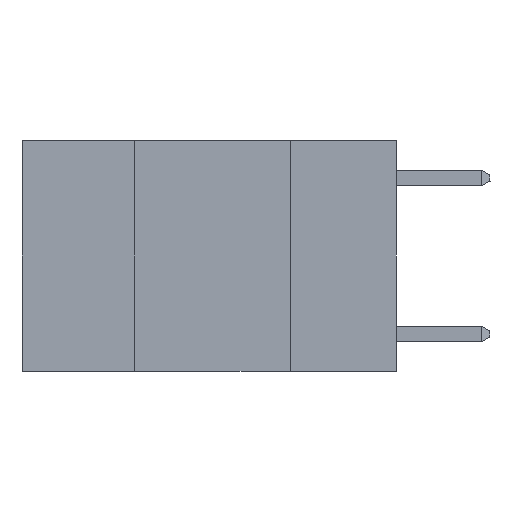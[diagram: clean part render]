
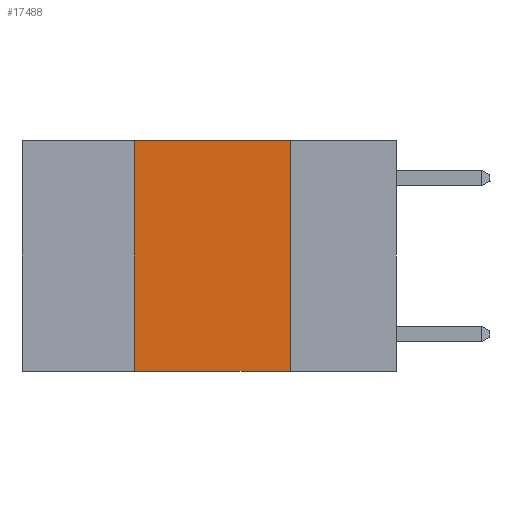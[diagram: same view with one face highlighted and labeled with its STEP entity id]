
A CAD part, left-side view. The second image highlights one B-rep face of the part: STEP entity #17488.
In plain terms, the highlighted planar face has unit normal (-1, 0, 0).
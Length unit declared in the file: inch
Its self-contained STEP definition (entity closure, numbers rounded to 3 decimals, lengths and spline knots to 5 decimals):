
#392 = LINE ( 'NONE', #9788, #3777 ) ;
#602 = PLANE ( 'NONE',  #5890 ) ;
#2267 = DIRECTION ( 'NONE',  ( 0., 0., -1. ) ) ;
#3777 = VECTOR ( 'NONE', #11441, 39.37008 ) ;
#4292 = LINE ( 'NONE', #11840, #12567 ) ;
#4605 = CARTESIAN_POINT ( 'NONE',  ( 0., 0.42, 0. ) ) ;
#5890 = AXIS2_PLACEMENT_3D ( 'NONE', #15410, #12222, #2267 ) ;
#6074 = LINE ( 'NONE', #7204, #8950 ) ;
#6252 = EDGE_LOOP ( 'NONE', ( #10040, #10189, #10348, #10384 ) ) ;
#7204 = CARTESIAN_POINT ( 'NONE',  ( 0., 0.17, 0. ) ) ;
#7452 = EDGE_CURVE ( 'NONE', #16539, #14102, #392, .T. ) ;
#8306 = CARTESIAN_POINT ( 'NONE',  ( 0., 0.17, -0.37 ) ) ;
#8326 = EDGE_CURVE ( 'NONE', #13543, #9636, #4292, .T. ) ;
#8492 = EDGE_CURVE ( 'NONE', #14102, #9636, #6074, .T. ) ;
#8708 = EDGE_CURVE ( 'NONE', #13543, #16539, #20873, .T. ) ;
#8950 = VECTOR ( 'NONE', #15447, 39.37008 ) ;
#9636 = VERTEX_POINT ( 'NONE', #8306 ) ;
#9788 = CARTESIAN_POINT ( 'NONE',  ( 0., 0.6, 0. ) ) ;
#9900 = CARTESIAN_POINT ( 'NONE',  ( 0., 0.42, -0.37 ) ) ;
#10040 = ORIENTED_EDGE ( 'NONE', *, *, #8492, .F. ) ;
#10189 = ORIENTED_EDGE ( 'NONE', *, *, #7452, .F. ) ;
#10348 = ORIENTED_EDGE ( 'NONE', *, *, #8708, .F. ) ;
#10384 = ORIENTED_EDGE ( 'NONE', *, *, #8326, .T. ) ;
#11441 = DIRECTION ( 'NONE',  ( 0., -1., 0. ) ) ;
#11840 = CARTESIAN_POINT ( 'NONE',  ( 0., 0.6, -0.37 ) ) ;
#12222 = DIRECTION ( 'NONE',  ( 1., 0., 0. ) ) ;
#12567 = VECTOR ( 'NONE', #13465, 39.37008 ) ;
#13465 = DIRECTION ( 'NONE',  ( 0., -1., 0. ) ) ;
#13543 = VERTEX_POINT ( 'NONE', #9900 ) ;
#14102 = VERTEX_POINT ( 'NONE', #14523 ) ;
#14523 = CARTESIAN_POINT ( 'NONE',  ( 0., 0.17, 0. ) ) ;
#14579 = FACE_OUTER_BOUND ( 'NONE', #6252, .T. ) ;
#15410 = CARTESIAN_POINT ( 'NONE',  ( 0., 0.6, 0. ) ) ;
#15447 = DIRECTION ( 'NONE',  ( 0., 0., -1. ) ) ;
#16539 = VERTEX_POINT ( 'NONE', #17941 ) ;
#17327 = VECTOR ( 'NONE', #17679, 39.37008 ) ;
#17488 = ADVANCED_FACE ( 'NONE', ( #14579 ), #602, .F. ) ;
#17679 = DIRECTION ( 'NONE',  ( 0., 0., 1. ) ) ;
#17941 = CARTESIAN_POINT ( 'NONE',  ( 0., 0.42, 0. ) ) ;
#20873 = LINE ( 'NONE', #4605, #17327 ) ;
